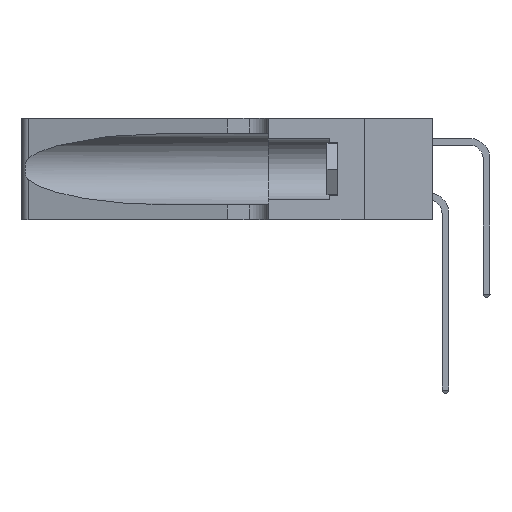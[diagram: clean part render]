
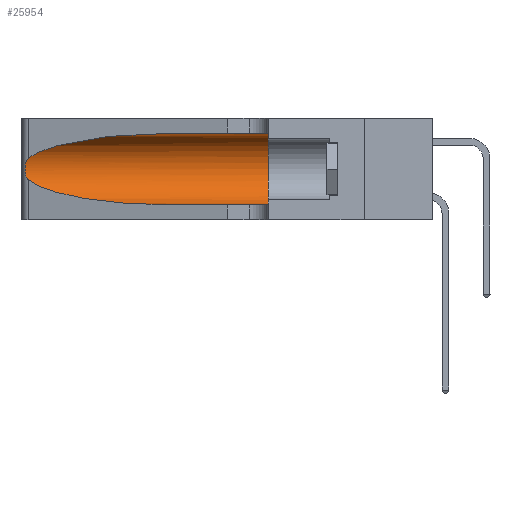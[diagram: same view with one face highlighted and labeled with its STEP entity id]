
A CAD part, left-side view. The second image highlights one B-rep face of the part: STEP entity #25954.
In plain terms, the highlighted cylindrical face has radius 3.308 mm (diameter 6.617 mm), a partial arc.
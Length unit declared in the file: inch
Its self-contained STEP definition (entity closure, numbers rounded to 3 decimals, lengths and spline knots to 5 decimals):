
#595 = ORIENTED_EDGE ( 'NONE', *, *, #9039, .F. ) ;
#852 = VECTOR ( 'NONE', #4676, 39.37008 ) ;
#1078 = ORIENTED_EDGE ( 'NONE', *, *, #25092, .T. ) ;
#1193 = CARTESIAN_POINT ( 'NONE',  ( 0.25789, 1.23486, 0.15765 ) ) ;
#1340 = VECTOR ( 'NONE', #13770, 39.37008 ) ;
#1352 = CARTESIAN_POINT ( 'NONE',  ( 0.1305, 0.72297, 0.05475 ) ) ;
#2371 = CYLINDRICAL_SURFACE ( 'NONE', #16287, 0.13025 ) ;
#2976 = VERTEX_POINT ( 'NONE', #8779 ) ;
#3206 = FACE_OUTER_BOUND ( 'NONE', #28893, .T. ) ;
#3849 = CARTESIAN_POINT ( 'NONE',  ( 0.25555, 1.22993, 0.14849 ) ) ;
#4094 = VERTEX_POINT ( 'NONE', #6727 ) ;
#4324 = CARTESIAN_POINT ( 'NONE',  ( 0.1305, 0.72297, 0.05475 ) ) ;
#4458 = CARTESIAN_POINT ( 'NONE',  ( 0.1305, 0.35, 0.31525 ) ) ;
#4676 = DIRECTION ( 'NONE',  ( 0., -1., 0. ) ) ;
#4884 = ORIENTED_EDGE ( 'NONE', *, *, #15787, .T. ) ;
#5234 =( BOUNDED_CURVE ( )  B_SPLINE_CURVE ( 3, ( #14629, #29615, #19651, #4324 ),
 .UNSPECIFIED., .F., .F. ) 
 B_SPLINE_CURVE_WITH_KNOTS ( ( 4, 4 ),
 ( 3.44316, 4.71239 ),
 .UNSPECIFIED. ) 
 CURVE ( )  GEOMETRIC_REPRESENTATION_ITEM ( )  RATIONAL_B_SPLINE_CURVE ( ( 1., 0.87, 0.87, 1. ) ) 
 REPRESENTATION_ITEM ( '' )  );
#6299 = CARTESIAN_POINT ( 'NONE',  ( 0.25555, 1.22994, 0.2215 ) ) ;
#6727 = CARTESIAN_POINT ( 'NONE',  ( 0.1305, 0.35, 0.05475 ) ) ;
#7506 = CIRCLE ( 'NONE', #17081, 0.13025 ) ;
#7677 = CARTESIAN_POINT ( 'NONE',  ( 0.1305, 1.61858, 0.185 ) ) ;
#7990 = VERTEX_POINT ( 'NONE', #13377 ) ;
#8779 = CARTESIAN_POINT ( 'NONE',  ( 0.25487, 1.22718, 0.22369 ) ) ;
#8918 = CARTESIAN_POINT ( 'NONE',  ( 0.25787, 1.23484, 0.2124 ) ) ;
#9039 = EDGE_CURVE ( 'NONE', #7990, #20554, #27183, .T. ) ;
#9395 = ORIENTED_EDGE ( 'NONE', *, *, #29304, .T. ) ;
#11280 = B_SPLINE_CURVE_WITH_KNOTS ( 'NONE', 3,
 ( #21593, #6299, #24073, #8918, #26602, #11554, #29138, #14155, #31608, #16677, #1193, #19186, #3849, #21700 ),
 .UNSPECIFIED., .F., .F.,
 ( 4, 2, 2, 2, 2, 2, 4 ),
 ( 0., 0.00027, 0.00053, 0.00107, 0.0016, 0.00187, 0.00214 ),
 .UNSPECIFIED. ) ;
#11554 = CARTESIAN_POINT ( 'NONE',  ( 0.26018, 1.23835, 0.19895 ) ) ;
#12329 =( BOUNDED_CURVE ( )  B_SPLINE_CURVE ( 3, ( #26980, #29513, #31975, #17037 ),
 .UNSPECIFIED., .F., .F. ) 
 B_SPLINE_CURVE_WITH_KNOTS ( ( 4, 4 ),
 ( 1.5708, 2.84003 ),
 .UNSPECIFIED. ) 
 CURVE ( )  GEOMETRIC_REPRESENTATION_ITEM ( )  RATIONAL_B_SPLINE_CURVE ( ( 1., 0.87, 0.87, 1. ) ) 
 REPRESENTATION_ITEM ( '' )  );
#12684 = DIRECTION ( 'NONE',  ( 0., 1., 0. ) ) ;
#12913 = DIRECTION ( 'NONE',  ( 0., 0., -1. ) ) ;
#13377 = CARTESIAN_POINT ( 'NONE',  ( 0.1305, 0.72297, 0.31525 ) ) ;
#13418 = ORIENTED_EDGE ( 'NONE', *, *, #13811, .F. ) ;
#13551 = EDGE_CURVE ( 'NONE', #2976, #22760, #11280, .T. ) ;
#13770 = DIRECTION ( 'NONE',  ( 0., -1., 0. ) ) ;
#13811 = EDGE_CURVE ( 'NONE', #20554, #4094, #7506, .T. ) ;
#14155 = CARTESIAN_POINT ( 'NONE',  ( 0.26075, 1.23896, 0.178 ) ) ;
#14629 = CARTESIAN_POINT ( 'NONE',  ( 0.25487, 1.22718, 0.14631 ) ) ;
#15147 = LINE ( 'NONE', #15508, #1340 ) ;
#15508 = CARTESIAN_POINT ( 'NONE',  ( 0.1305, 1.61858, 0.05475 ) ) ;
#15787 = EDGE_CURVE ( 'NONE', #22760, #20975, #5234, .T. ) ;
#16287 = AXIS2_PLACEMENT_3D ( 'NONE', #7677, #25397, #12913 ) ;
#16677 = CARTESIAN_POINT ( 'NONE',  ( 0.25856, 1.23593, 0.16098 ) ) ;
#17037 = CARTESIAN_POINT ( 'NONE',  ( 0.25487, 1.22718, 0.22369 ) ) ;
#17081 = AXIS2_PLACEMENT_3D ( 'NONE', #27701, #12684, #30213 ) ;
#19186 = CARTESIAN_POINT ( 'NONE',  ( 0.25639, 1.23186, 0.15144 ) ) ;
#19651 = CARTESIAN_POINT ( 'NONE',  ( 0.18966, 0.96281, 0.05475 ) ) ;
#20004 = CARTESIAN_POINT ( 'NONE',  ( 0.1305, 1.61858, 0.31525 ) ) ;
#20554 = VERTEX_POINT ( 'NONE', #4458 ) ;
#20975 = VERTEX_POINT ( 'NONE', #1352 ) ;
#21593 = CARTESIAN_POINT ( 'NONE',  ( 0.25487, 1.22718, 0.22369 ) ) ;
#21700 = CARTESIAN_POINT ( 'NONE',  ( 0.25487, 1.22718, 0.14631 ) ) ;
#22760 = VERTEX_POINT ( 'NONE', #25573 ) ;
#24073 = CARTESIAN_POINT ( 'NONE',  ( 0.25639, 1.23184, 0.21858 ) ) ;
#24542 = ORIENTED_EDGE ( 'NONE', *, *, #13551, .T. ) ;
#25092 = EDGE_CURVE ( 'NONE', #7990, #2976, #12329, .T. ) ;
#25397 = DIRECTION ( 'NONE',  ( 0., -1., 0. ) ) ;
#25573 = CARTESIAN_POINT ( 'NONE',  ( 0.25487, 1.22718, 0.14631 ) ) ;
#25954 = ADVANCED_FACE ( 'NONE', ( #3206 ), #2371, .F. ) ;
#26602 = CARTESIAN_POINT ( 'NONE',  ( 0.25854, 1.2359, 0.20912 ) ) ;
#26980 = CARTESIAN_POINT ( 'NONE',  ( 0.1305, 0.72297, 0.31525 ) ) ;
#27183 = LINE ( 'NONE', #20004, #852 ) ;
#27701 = CARTESIAN_POINT ( 'NONE',  ( 0.1305, 0.35, 0.185 ) ) ;
#28893 = EDGE_LOOP ( 'NONE', ( #1078, #24542, #4884, #9395, #13418, #595 ) ) ;
#29138 = CARTESIAN_POINT ( 'NONE',  ( 0.26075, 1.23896, 0.19203 ) ) ;
#29304 = EDGE_CURVE ( 'NONE', #20975, #4094, #15147, .T. ) ;
#29513 = CARTESIAN_POINT ( 'NONE',  ( 0.18966, 0.96281, 0.31525 ) ) ;
#29615 = CARTESIAN_POINT ( 'NONE',  ( 0.2373, 1.15595, 0.08982 ) ) ;
#30213 = DIRECTION ( 'NONE',  ( 0., 0., 1. ) ) ;
#31608 = CARTESIAN_POINT ( 'NONE',  ( 0.26017, 1.23833, 0.17102 ) ) ;
#31975 = CARTESIAN_POINT ( 'NONE',  ( 0.2373, 1.15595, 0.28018 ) ) ;
